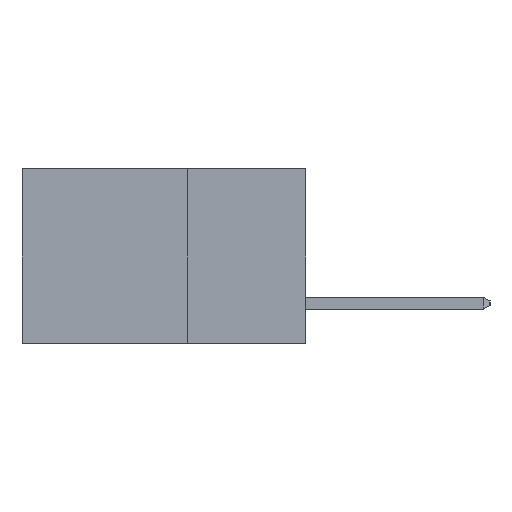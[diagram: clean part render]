
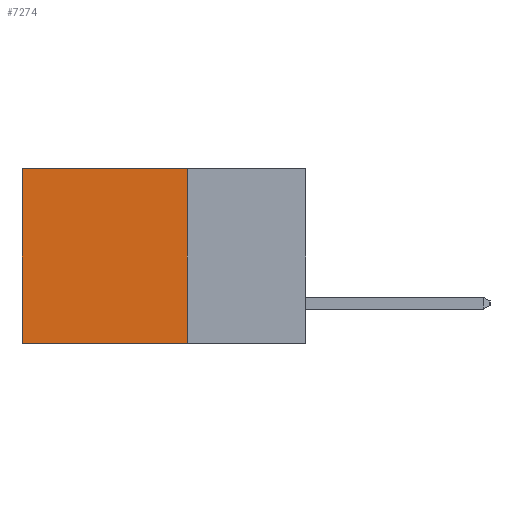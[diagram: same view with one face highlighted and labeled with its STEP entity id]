
A CAD part, left-side view. The second image highlights one B-rep face of the part: STEP entity #7274.
In plain terms, the highlighted planar face has unit normal (-1, 0, 0).
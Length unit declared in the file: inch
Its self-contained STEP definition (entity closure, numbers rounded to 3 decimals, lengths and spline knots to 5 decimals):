
#409 = DIRECTION ( 'NONE',  ( 0., 1., 0. ) ) ;
#423 = ORIENTED_EDGE ( 'NONE', *, *, #1273, .F. ) ;
#650 = LINE ( 'NONE', #7086, #4183 ) ;
#1273 = EDGE_CURVE ( 'NONE', #2100, #3192, #3917, .T. ) ;
#1323 = EDGE_CURVE ( 'NONE', #5319, #5344, #7313, .T. ) ;
#1331 = ORIENTED_EDGE ( 'NONE', *, *, #1323, .T. ) ;
#1423 = CARTESIAN_POINT ( 'NONE',  ( 0.2615, 0.6, -0.37 ) ) ;
#1818 = FACE_OUTER_BOUND ( 'NONE', #3466, .T. ) ;
#2077 = CARTESIAN_POINT ( 'NONE',  ( 0.2615, 0.25, -0.37 ) ) ;
#2100 = VERTEX_POINT ( 'NONE', #4060 ) ;
#2107 = EDGE_CURVE ( 'NONE', #3192, #5344, #6512, .T. ) ;
#2836 = CARTESIAN_POINT ( 'NONE',  ( 0.2615, 0.6, -0.37 ) ) ;
#2931 = DIRECTION ( 'NONE',  ( 0., 0., -1. ) ) ;
#3151 = CARTESIAN_POINT ( 'NONE',  ( 0.2615, 0.25, -0.37 ) ) ;
#3157 = DIRECTION ( 'NONE',  ( 0., 0., -1. ) ) ;
#3192 = VERTEX_POINT ( 'NONE', #2077 ) ;
#3466 = EDGE_LOOP ( 'NONE', ( #1331, #5909, #423, #4853 ) ) ;
#3553 = DIRECTION ( 'NONE',  ( 0., 1., 0. ) ) ;
#3627 = CARTESIAN_POINT ( 'NONE',  ( 0.2615, 0.25, -0.37 ) ) ;
#3917 = LINE ( 'NONE', #3151, #9226 ) ;
#4060 = CARTESIAN_POINT ( 'NONE',  ( 0.2615, 0.25, 0. ) ) ;
#4183 = VECTOR ( 'NONE', #409, 39.37008 ) ;
#4196 = DIRECTION ( 'NONE',  ( 0., 0., -1. ) ) ;
#4729 = AXIS2_PLACEMENT_3D ( 'NONE', #4907, #8510, #4196 ) ;
#4819 = VECTOR ( 'NONE', #3553, 39.37008 ) ;
#4853 = ORIENTED_EDGE ( 'NONE', *, *, #5155, .T. ) ;
#4907 = CARTESIAN_POINT ( 'NONE',  ( 0.2615, 0.25, -0.37 ) ) ;
#5155 = EDGE_CURVE ( 'NONE', #2100, #5319, #650, .T. ) ;
#5188 = VECTOR ( 'NONE', #2931, 39.37008 ) ;
#5319 = VERTEX_POINT ( 'NONE', #9377 ) ;
#5344 = VERTEX_POINT ( 'NONE', #1423 ) ;
#5909 = ORIENTED_EDGE ( 'NONE', *, *, #2107, .F. ) ;
#6512 = LINE ( 'NONE', #3627, #4819 ) ;
#7086 = CARTESIAN_POINT ( 'NONE',  ( 0.2615, 0.25, 0. ) ) ;
#7274 = ADVANCED_FACE ( 'NONE', ( #1818 ), #7781, .F. ) ;
#7313 = LINE ( 'NONE', #2836, #5188 ) ;
#7781 = PLANE ( 'NONE',  #4729 ) ;
#8510 = DIRECTION ( 'NONE',  ( 1., 0., 0. ) ) ;
#9226 = VECTOR ( 'NONE', #3157, 39.37008 ) ;
#9377 = CARTESIAN_POINT ( 'NONE',  ( 0.2615, 0.6, 0. ) ) ;
